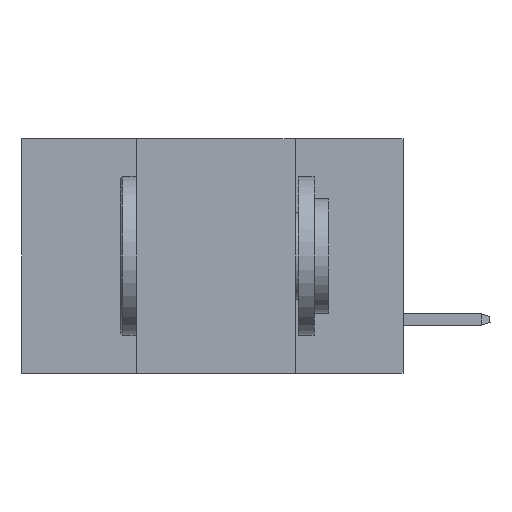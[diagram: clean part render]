
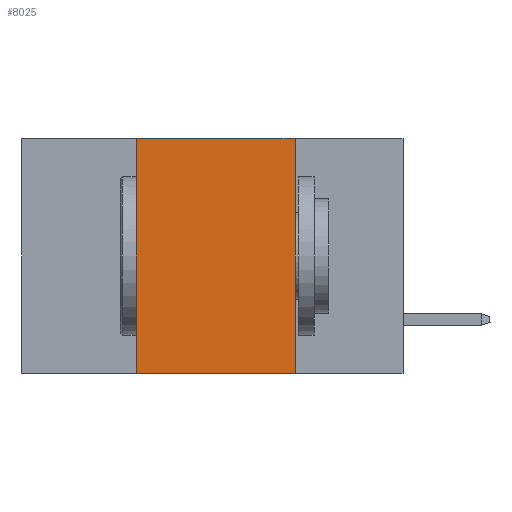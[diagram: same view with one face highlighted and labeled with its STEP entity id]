
A CAD part, left-side view. The second image highlights one B-rep face of the part: STEP entity #8025.
In plain terms, the highlighted planar face has unit normal (-1, 0, 0).
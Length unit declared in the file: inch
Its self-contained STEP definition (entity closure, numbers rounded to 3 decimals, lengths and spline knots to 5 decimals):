
#107 = CARTESIAN_POINT ( 'NONE',  ( 0., 0.17, 0. ) ) ;
#201 = DIRECTION ( 'NONE',  ( 0., -1., 0. ) ) ;
#342 = DIRECTION ( 'NONE',  ( 0., -1., 0. ) ) ;
#503 = EDGE_CURVE ( 'NONE', #10011, #21422, #17342, .T. ) ;
#715 = DIRECTION ( 'NONE',  ( 0., 0., 1. ) ) ;
#1177 = CARTESIAN_POINT ( 'NONE',  ( 0., 0.6, 0. ) ) ;
#2123 = CARTESIAN_POINT ( 'NONE',  ( 0., 0.6, 0. ) ) ;
#2236 = VECTOR ( 'NONE', #715, 39.37008 ) ;
#2745 = FACE_OUTER_BOUND ( 'NONE', #15455, .T. ) ;
#3770 = LINE ( 'NONE', #15430, #6254 ) ;
#3846 = CARTESIAN_POINT ( 'NONE',  ( 0., 0.42, 0. ) ) ;
#4351 = EDGE_CURVE ( 'NONE', #21422, #12956, #8499, .T. ) ;
#4546 = CARTESIAN_POINT ( 'NONE',  ( 0., 0.42, -0.37 ) ) ;
#6254 = VECTOR ( 'NONE', #201, 39.37008 ) ;
#6723 = CARTESIAN_POINT ( 'NONE',  ( 0., 0.17, 0. ) ) ;
#8025 = ADVANCED_FACE ( 'NONE', ( #2745 ), #19620, .F. ) ;
#8499 = LINE ( 'NONE', #6723, #20068 ) ;
#8960 = VERTEX_POINT ( 'NONE', #4546 ) ;
#10011 = VERTEX_POINT ( 'NONE', #11922 ) ;
#11922 = CARTESIAN_POINT ( 'NONE',  ( 0., 0.42, 0. ) ) ;
#12204 = ORIENTED_EDGE ( 'NONE', *, *, #17102, .T. ) ;
#12318 = ORIENTED_EDGE ( 'NONE', *, *, #14139, .F. ) ;
#12695 = VECTOR ( 'NONE', #342, 39.37008 ) ;
#12956 = VERTEX_POINT ( 'NONE', #15004 ) ;
#13101 = AXIS2_PLACEMENT_3D ( 'NONE', #1177, #21516, #18169 ) ;
#13476 = DIRECTION ( 'NONE',  ( 0., 0., -1. ) ) ;
#14139 = EDGE_CURVE ( 'NONE', #8960, #10011, #14259, .T. ) ;
#14259 = LINE ( 'NONE', #3846, #2236 ) ;
#15004 = CARTESIAN_POINT ( 'NONE',  ( 0., 0.17, -0.37 ) ) ;
#15430 = CARTESIAN_POINT ( 'NONE',  ( 0., 0.6, -0.37 ) ) ;
#15455 = EDGE_LOOP ( 'NONE', ( #19199, #18426, #12318, #12204 ) ) ;
#17102 = EDGE_CURVE ( 'NONE', #8960, #12956, #3770, .T. ) ;
#17342 = LINE ( 'NONE', #2123, #12695 ) ;
#18169 = DIRECTION ( 'NONE',  ( 0., 0., -1. ) ) ;
#18426 = ORIENTED_EDGE ( 'NONE', *, *, #503, .F. ) ;
#19199 = ORIENTED_EDGE ( 'NONE', *, *, #4351, .F. ) ;
#19620 = PLANE ( 'NONE',  #13101 ) ;
#20068 = VECTOR ( 'NONE', #13476, 39.37008 ) ;
#21422 = VERTEX_POINT ( 'NONE', #107 ) ;
#21516 = DIRECTION ( 'NONE',  ( 1., 0., 0. ) ) ;
